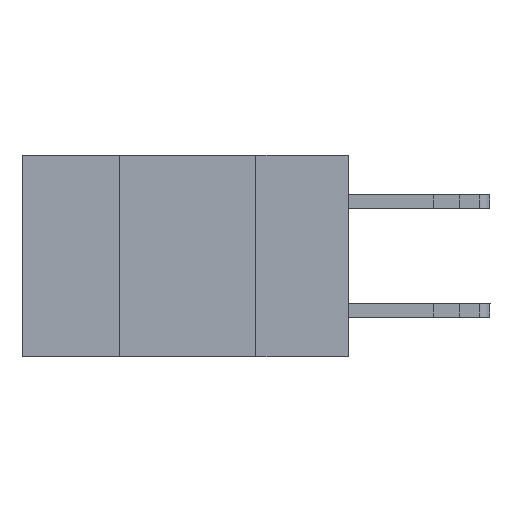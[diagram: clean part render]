
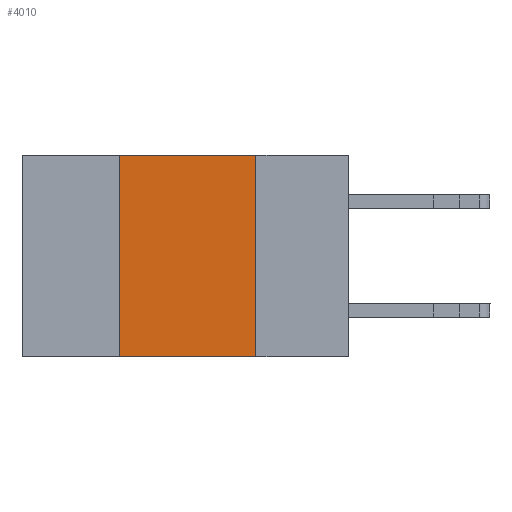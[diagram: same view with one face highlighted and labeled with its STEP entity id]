
A CAD part, left-side view. The second image highlights one B-rep face of the part: STEP entity #4010.
In plain terms, the highlighted planar face has unit normal (-1, 0, 0).
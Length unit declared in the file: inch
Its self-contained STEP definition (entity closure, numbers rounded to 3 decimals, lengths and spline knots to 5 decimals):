
#247 = PLANE ( 'NONE',  #6849 ) ;
#298 = DIRECTION ( 'NONE',  ( 0., 0., -1. ) ) ;
#345 = ORIENTED_EDGE ( 'NONE', *, *, #7953, .F. ) ;
#359 = CARTESIAN_POINT ( 'NONE',  ( 0., 0.6, 0. ) ) ;
#1327 = EDGE_CURVE ( 'NONE', #4730, #10602, #10850, .T. ) ;
#1666 = VECTOR ( 'NONE', #4599, 39.37008 ) ;
#2180 = DIRECTION ( 'NONE',  ( 0., 0., -1. ) ) ;
#2329 = CARTESIAN_POINT ( 'NONE',  ( 0., 0.6, 0. ) ) ;
#2408 = EDGE_LOOP ( 'NONE', ( #345, #5565, #7852, #10540 ) ) ;
#2637 = LINE ( 'NONE', #6173, #5686 ) ;
#3568 = CARTESIAN_POINT ( 'NONE',  ( 0., 0.42, 0. ) ) ;
#3754 = LINE ( 'NONE', #5160, #11493 ) ;
#4010 = ADVANCED_FACE ( 'NONE', ( #12828 ), #247, .F. ) ;
#4366 = DIRECTION ( 'NONE',  ( 1., 0., 0. ) ) ;
#4599 = DIRECTION ( 'NONE',  ( 0., 0., 1. ) ) ;
#4730 = VERTEX_POINT ( 'NONE', #9679 ) ;
#5160 = CARTESIAN_POINT ( 'NONE',  ( 0., 0.17, 0. ) ) ;
#5565 = ORIENTED_EDGE ( 'NONE', *, *, #1327, .F. ) ;
#5686 = VECTOR ( 'NONE', #8433, 39.37008 ) ;
#5837 = LINE ( 'NONE', #3568, #1666 ) ;
#6102 = CARTESIAN_POINT ( 'NONE',  ( 0., 0.17, -0.37 ) ) ;
#6173 = CARTESIAN_POINT ( 'NONE',  ( 0., 0.6, -0.37 ) ) ;
#6542 = VECTOR ( 'NONE', #6575, 39.37008 ) ;
#6571 = VERTEX_POINT ( 'NONE', #13195 ) ;
#6575 = DIRECTION ( 'NONE',  ( 0., -1., 0. ) ) ;
#6849 = AXIS2_PLACEMENT_3D ( 'NONE', #2329, #4366, #298 ) ;
#6971 = CARTESIAN_POINT ( 'NONE',  ( 0., 0.17, 0. ) ) ;
#7852 = ORIENTED_EDGE ( 'NONE', *, *, #8923, .F. ) ;
#7953 = EDGE_CURVE ( 'NONE', #10602, #12530, #3754, .T. ) ;
#8433 = DIRECTION ( 'NONE',  ( 0., -1., 0. ) ) ;
#8923 = EDGE_CURVE ( 'NONE', #6571, #4730, #5837, .T. ) ;
#9679 = CARTESIAN_POINT ( 'NONE',  ( 0., 0.42, 0. ) ) ;
#10540 = ORIENTED_EDGE ( 'NONE', *, *, #11801, .T. ) ;
#10602 = VERTEX_POINT ( 'NONE', #6971 ) ;
#10850 = LINE ( 'NONE', #359, #6542 ) ;
#11493 = VECTOR ( 'NONE', #2180, 39.37008 ) ;
#11801 = EDGE_CURVE ( 'NONE', #6571, #12530, #2637, .T. ) ;
#12530 = VERTEX_POINT ( 'NONE', #6102 ) ;
#12828 = FACE_OUTER_BOUND ( 'NONE', #2408, .T. ) ;
#13195 = CARTESIAN_POINT ( 'NONE',  ( 0., 0.42, -0.37 ) ) ;
